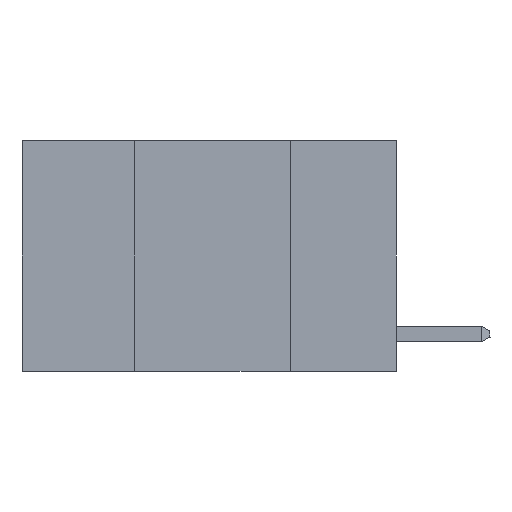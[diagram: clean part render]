
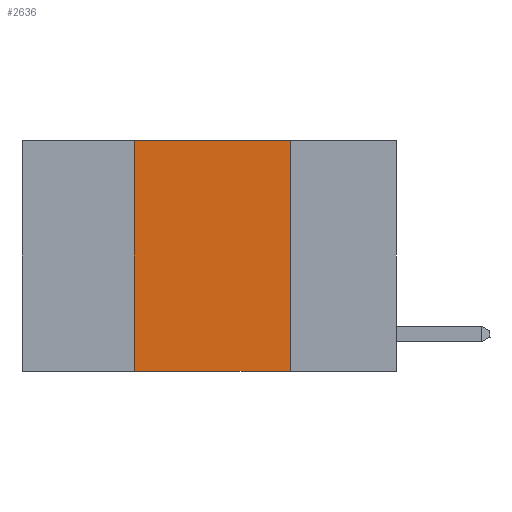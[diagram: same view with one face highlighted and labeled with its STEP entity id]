
A CAD part, left-side view. The second image highlights one B-rep face of the part: STEP entity #2636.
In plain terms, the highlighted planar face has unit normal (-1, 0, 0).
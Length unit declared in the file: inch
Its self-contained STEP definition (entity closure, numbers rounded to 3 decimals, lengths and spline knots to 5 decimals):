
#476 = PLANE ( 'NONE',  #16627 ) ;
#812 = VERTEX_POINT ( 'NONE', #20663 ) ;
#864 = VERTEX_POINT ( 'NONE', #1963 ) ;
#970 = ORIENTED_EDGE ( 'NONE', *, *, #6340, .F. ) ;
#1001 = CARTESIAN_POINT ( 'NONE',  ( 0., 0.17, 0. ) ) ;
#1596 = CARTESIAN_POINT ( 'NONE',  ( 0., 0.42, 0. ) ) ;
#1704 = VERTEX_POINT ( 'NONE', #1596 ) ;
#1963 = CARTESIAN_POINT ( 'NONE',  ( 0., 0.17, 0. ) ) ;
#2636 = ADVANCED_FACE ( 'NONE', ( #10152 ), #476, .F. ) ;
#2995 = VERTEX_POINT ( 'NONE', #16943 ) ;
#3555 = VECTOR ( 'NONE', #13005, 39.37008 ) ;
#3771 = LINE ( 'NONE', #6300, #12410 ) ;
#3931 = DIRECTION ( 'NONE',  ( 0., 0., -1. ) ) ;
#4747 = ORIENTED_EDGE ( 'NONE', *, *, #10423, .F. ) ;
#5792 = EDGE_LOOP ( 'NONE', ( #4747, #970, #14189, #21458 ) ) ;
#6300 = CARTESIAN_POINT ( 'NONE',  ( 0., 0.42, 0. ) ) ;
#6340 = EDGE_CURVE ( 'NONE', #1704, #864, #17370, .T. ) ;
#8020 = DIRECTION ( 'NONE',  ( 0., 0., 1. ) ) ;
#9376 = LINE ( 'NONE', #1001, #19150 ) ;
#10152 = FACE_OUTER_BOUND ( 'NONE', #5792, .T. ) ;
#10423 = EDGE_CURVE ( 'NONE', #864, #2995, #9376, .T. ) ;
#12410 = VECTOR ( 'NONE', #8020, 39.37008 ) ;
#12525 = CARTESIAN_POINT ( 'NONE',  ( 0., 0.6, 0. ) ) ;
#13005 = DIRECTION ( 'NONE',  ( 0., -1., 0. ) ) ;
#13038 = DIRECTION ( 'NONE',  ( 0., -1., 0. ) ) ;
#13509 = LINE ( 'NONE', #21637, #21592 ) ;
#14189 = ORIENTED_EDGE ( 'NONE', *, *, #21296, .F. ) ;
#14303 = DIRECTION ( 'NONE',  ( 1., 0., 0. ) ) ;
#15551 = EDGE_CURVE ( 'NONE', #812, #2995, #13509, .T. ) ;
#16627 = AXIS2_PLACEMENT_3D ( 'NONE', #12525, #14303, #3931 ) ;
#16943 = CARTESIAN_POINT ( 'NONE',  ( 0., 0.17, -0.37 ) ) ;
#17370 = LINE ( 'NONE', #21612, #3555 ) ;
#18308 = DIRECTION ( 'NONE',  ( 0., 0., -1. ) ) ;
#19150 = VECTOR ( 'NONE', #18308, 39.37008 ) ;
#20663 = CARTESIAN_POINT ( 'NONE',  ( 0., 0.42, -0.37 ) ) ;
#21296 = EDGE_CURVE ( 'NONE', #812, #1704, #3771, .T. ) ;
#21458 = ORIENTED_EDGE ( 'NONE', *, *, #15551, .T. ) ;
#21592 = VECTOR ( 'NONE', #13038, 39.37008 ) ;
#21612 = CARTESIAN_POINT ( 'NONE',  ( 0., 0.6, 0. ) ) ;
#21637 = CARTESIAN_POINT ( 'NONE',  ( 0., 0.6, -0.37 ) ) ;
